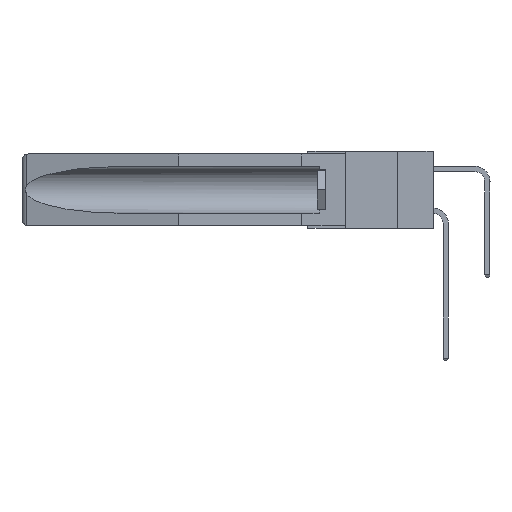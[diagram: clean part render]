
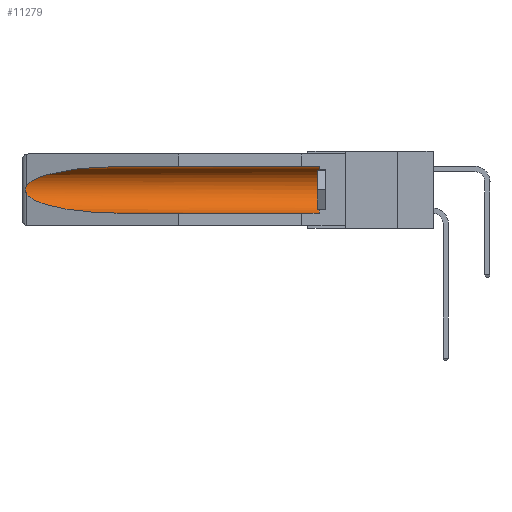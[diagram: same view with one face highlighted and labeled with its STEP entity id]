
A CAD part, left-side view. The second image highlights one B-rep face of the part: STEP entity #11279.
In plain terms, the highlighted cylindrical face has radius 2.857 mm (diameter 5.715 mm), a partial arc.
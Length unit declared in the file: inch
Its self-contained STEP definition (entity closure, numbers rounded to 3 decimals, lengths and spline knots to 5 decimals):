
#793 = CARTESIAN_POINT ( 'NONE',  ( 0.25451, 1.48313, -0.24835 ) ) ;
#2353 = VERTEX_POINT ( 'NONE', #27173 ) ;
#3383 = CARTESIAN_POINT ( 'NONE',  ( 0.21114, 1.30732, -0.284 ) ) ;
#3558 = EDGE_CURVE ( 'NONE', #23451, #8986, #9928, .T. ) ;
#3747 = CARTESIAN_POINT ( 'NONE',  ( 0.155, -0.30754, -0.284 ) ) ;
#4488 = EDGE_CURVE ( 'NONE', #2353, #23451, #8291, .T. ) ;
#4581 = ORIENTED_EDGE ( 'NONE', *, *, #5084, .T. ) ;
#5084 = EDGE_CURVE ( 'NONE', #24807, #2353, #7841, .T. ) ;
#5614 = LINE ( 'NONE', #3747, #25224 ) ;
#5790 = CYLINDRICAL_SURFACE ( 'NONE', #18185, 0.1125 ) ;
#6022 = CARTESIAN_POINT ( 'NONE',  ( 0.26655, 1.53094, -0.18657 ) ) ;
#6795 = ORIENTED_EDGE ( 'NONE', *, *, #25765, .T. ) ;
#7841 = CIRCLE ( 'NONE', #10998, 0.1125 ) ;
#8291 = LINE ( 'NONE', #23452, #22706 ) ;
#8571 = CARTESIAN_POINT ( 'NONE',  ( 0.26597, 1.52961, -0.15275 ) ) ;
#8687 = CARTESIAN_POINT ( 'NONE',  ( 0.26537, 1.52718, -0.14972 ) ) ;
#8787 = CARTESIAN_POINT ( 'NONE',  ( 0.26537, 1.52718, -0.19328 ) ) ;
#8805 = CARTESIAN_POINT ( 'NONE',  ( 0.155, 1.07973, -0.059 ) ) ;
#8986 = VERTEX_POINT ( 'NONE', #15479 ) ;
#9918 = CARTESIAN_POINT ( 'NONE',  ( 0.155, 0.126, -0.284 ) ) ;
#9928 =( BOUNDED_CURVE ( )  B_SPLINE_CURVE ( 3, ( #8805, #11508, #21436, #8687 ),
 .UNSPECIFIED., .F., .F. ) 
 B_SPLINE_CURVE_WITH_KNOTS ( ( 4, 4 ),
 ( 4.71239, 6.08839 ),
 .UNSPECIFIED. ) 
 CURVE ( )  GEOMETRIC_REPRESENTATION_ITEM ( )  RATIONAL_B_SPLINE_CURVE ( ( 1., 0.848, 0.848, 1. ) ) 
 REPRESENTATION_ITEM ( '' )  );
#10375 = DIRECTION ( 'NONE',  ( 0., 1., 0. ) ) ;
#10582 = EDGE_CURVE ( 'NONE', #16583, #19763, #25316, .T. ) ;
#10940 = CARTESIAN_POINT ( 'NONE',  ( 0.26537, 1.52718, -0.14972 ) ) ;
#10998 = AXIS2_PLACEMENT_3D ( 'NONE', #28226, #22859, #20391 ) ;
#11166 = DIRECTION ( 'NONE',  ( 0., 1., 0. ) ) ;
#11274 = CARTESIAN_POINT ( 'NONE',  ( 0.2675, 1.53308, -0.16763 ) ) ;
#11279 = ADVANCED_FACE ( 'NONE', ( #31786 ), #5790, .F. ) ;
#11326 = EDGE_LOOP ( 'NONE', ( #31256, #6795, #23210, #11705, #4581, #11338 ) ) ;
#11338 = ORIENTED_EDGE ( 'NONE', *, *, #4488, .T. ) ;
#11508 = CARTESIAN_POINT ( 'NONE',  ( 0.21114, 1.30732, -0.059 ) ) ;
#11705 = ORIENTED_EDGE ( 'NONE', *, *, #23775, .F. ) ;
#13511 = CARTESIAN_POINT ( 'NONE',  ( 0.2675, 1.53308, -0.17534 ) ) ;
#13729 = CARTESIAN_POINT ( 'NONE',  ( 0.2673, 1.53269, -0.17917 ) ) ;
#15479 = CARTESIAN_POINT ( 'NONE',  ( 0.26537, 1.52718, -0.14972 ) ) ;
#15874 = CARTESIAN_POINT ( 'NONE',  ( 0.155, -0.30754, -0.1715 ) ) ;
#16210 = CARTESIAN_POINT ( 'NONE',  ( 0.26654, 1.53092, -0.15636 ) ) ;
#16583 = VERTEX_POINT ( 'NONE', #29093 ) ;
#18185 = AXIS2_PLACEMENT_3D ( 'NONE', #15874, #11166, #29028 ) ;
#19348 = DIRECTION ( 'NONE',  ( 0., 1., 0. ) ) ;
#19763 = VERTEX_POINT ( 'NONE', #22963 ) ;
#20391 = DIRECTION ( 'NONE',  ( 0., 0., 1. ) ) ;
#21214 = CARTESIAN_POINT ( 'NONE',  ( 0.155, 1.07973, -0.284 ) ) ;
#21436 = CARTESIAN_POINT ( 'NONE',  ( 0.25451, 1.48313, -0.09465 ) ) ;
#22706 = VECTOR ( 'NONE', #10375, 39.37008 ) ;
#22859 = DIRECTION ( 'NONE',  ( 0., -1., 0. ) ) ;
#22963 = CARTESIAN_POINT ( 'NONE',  ( 0.155, 1.07973, -0.284 ) ) ;
#23210 = ORIENTED_EDGE ( 'NONE', *, *, #10582, .T. ) ;
#23451 = VERTEX_POINT ( 'NONE', #30878 ) ;
#23452 = CARTESIAN_POINT ( 'NONE',  ( 0.155, -0.30754, -0.059 ) ) ;
#23775 = EDGE_CURVE ( 'NONE', #24807, #19763, #5614, .T. ) ;
#24807 = VERTEX_POINT ( 'NONE', #9918 ) ;
#25224 = VECTOR ( 'NONE', #19348, 39.37008 ) ;
#25316 =( BOUNDED_CURVE ( )  B_SPLINE_CURVE ( 3, ( #28821, #793, #3383, #21214 ),
 .UNSPECIFIED., .F., .T. ) 
 B_SPLINE_CURVE_WITH_KNOTS ( ( 4, 4 ),
 ( 0.1948, 1.5708 ),
 .UNSPECIFIED. ) 
 CURVE ( )  GEOMETRIC_REPRESENTATION_ITEM ( )  RATIONAL_B_SPLINE_CURVE ( ( 1., 0.848, 0.848, 1. ) ) 
 REPRESENTATION_ITEM ( '' )  );
#25765 = EDGE_CURVE ( 'NONE', #8986, #16583, #29185, .T. ) ;
#27173 = CARTESIAN_POINT ( 'NONE',  ( 0.155, 0.126, -0.059 ) ) ;
#28226 = CARTESIAN_POINT ( 'NONE',  ( 0.155, 0.126, -0.1715 ) ) ;
#28821 = CARTESIAN_POINT ( 'NONE',  ( 0.26537, 1.52718, -0.19328 ) ) ;
#29028 = DIRECTION ( 'NONE',  ( 0., 0., 1. ) ) ;
#29093 = CARTESIAN_POINT ( 'NONE',  ( 0.26537, 1.52718, -0.19328 ) ) ;
#29185 = B_SPLINE_CURVE_WITH_KNOTS ( 'NONE', 3,
 ( #10940, #8571, #16210, #31494, #11274, #13511, #13729, #6022, #31714, #8787 ),
 .UNSPECIFIED., .F., .F.,
 ( 4, 2, 2, 2, 4 ),
 ( 0., 0.00029, 0.00058, 0.00087, 0.00117 ),
 .UNSPECIFIED. ) ;
#30878 = CARTESIAN_POINT ( 'NONE',  ( 0.155, 1.07973, -0.059 ) ) ;
#31256 = ORIENTED_EDGE ( 'NONE', *, *, #3558, .T. ) ;
#31494 = CARTESIAN_POINT ( 'NONE',  ( 0.2673, 1.5327, -0.16383 ) ) ;
#31714 = CARTESIAN_POINT ( 'NONE',  ( 0.26597, 1.5296, -0.19026 ) ) ;
#31786 = FACE_OUTER_BOUND ( 'NONE', #11326, .T. ) ;
